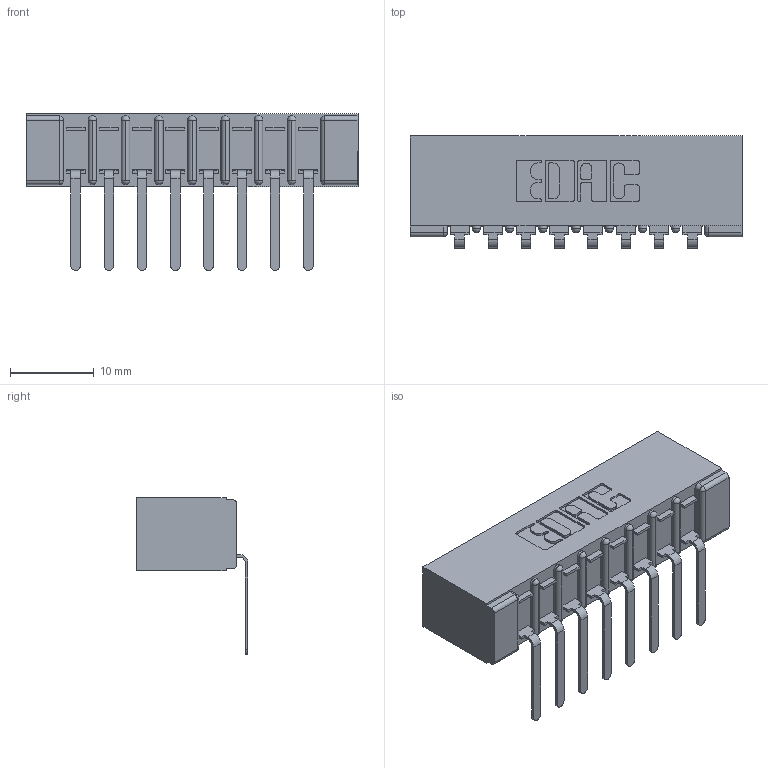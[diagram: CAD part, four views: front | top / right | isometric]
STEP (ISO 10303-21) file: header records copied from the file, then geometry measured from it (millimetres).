
FILE_DESCRIPTION (( 'STEP AP203' ), '1' );
FILE_NAME ('307-008-457-101.STEP', '2020-09-25T04:32:50', ( '' ), ( '' ), 'SwSTEP 2.0', 'SolidWorks 2020', '' );
FILE_SCHEMA (( 'CONFIG_CONTROL_DESIGN' ));
Length unit declared in the file: inch
Products named in the file (3): 307-008-457-101; 307 Part_No Mounting Lugs; 307-290-002_557
Assembly tree (9 placements, depth 2):
  307-008-457-101
    307 Part_No Mounting Lugs
    307-290-002_557  x8
Bounding box: 39.57 x 13.32 x 18.67 mm (x, y, z)
Volume: 2869.1 mm3; surface area: 5079.1 mm2
Topology: 9 solids, 9 shells, 743 faces, 2251 edges, 1474 vertices
Faces by surface type: plane 442, cylinder 283, sphere 18
Entity records: 11626 total; most frequent: CARTESIAN_POINT 1956, ORIENTED_EDGE 1946, DIRECTION 1915, EDGE_CURVE 973, VECTOR 729, LINE 729, VERTEX_POINT 634, AXIS2_PLACEMENT_3D 593
